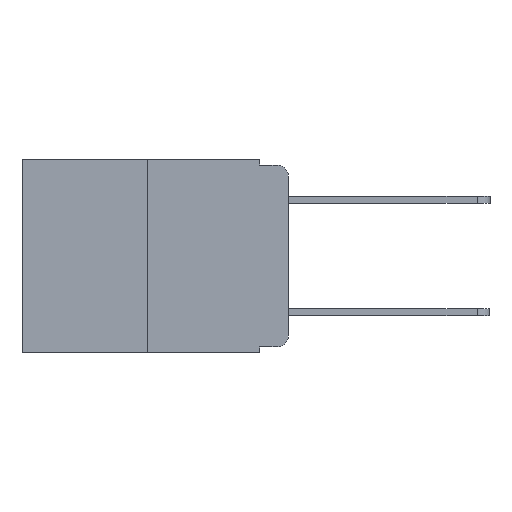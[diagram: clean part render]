
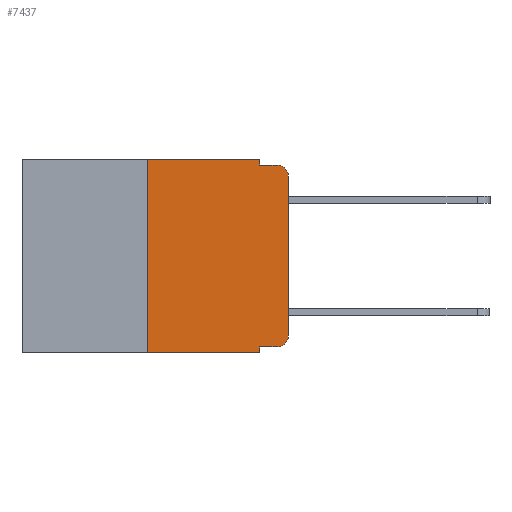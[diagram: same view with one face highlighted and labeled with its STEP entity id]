
A CAD part, left-side view. The second image highlights one B-rep face of the part: STEP entity #7437.
In plain terms, the highlighted planar face has unit normal (-1, 0, 0).
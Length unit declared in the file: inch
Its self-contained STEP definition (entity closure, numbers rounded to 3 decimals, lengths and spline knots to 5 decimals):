
#278 = PLANE ( 'NONE',  #517 ) ;
#517 = AXIS2_PLACEMENT_3D ( 'NONE', #5071, #8735, #3286 ) ;
#566 = ORIENTED_EDGE ( 'NONE', *, *, #10424, .F. ) ;
#667 = VECTOR ( 'NONE', #9923, 39.37008 ) ;
#811 = VERTEX_POINT ( 'NONE', #3382 ) ;
#826 = EDGE_CURVE ( 'NONE', #2921, #2967, #3867, .T. ) ;
#995 = EDGE_CURVE ( 'NONE', #6220, #811, #9644, .T. ) ;
#1177 = EDGE_CURVE ( 'NONE', #3896, #2921, #6181, .T. ) ;
#1472 = CIRCLE ( 'NONE', #2716, 0.02 ) ;
#1535 = CARTESIAN_POINT ( 'NONE',  ( 0., 0.051, -0.333 ) ) ;
#1595 = VERTEX_POINT ( 'NONE', #4728 ) ;
#1749 = EDGE_CURVE ( 'NONE', #9573, #2967, #1472, .T. ) ;
#1868 = ORIENTED_EDGE ( 'NONE', *, *, #7618, .T. ) ;
#2366 = LINE ( 'NONE', #7528, #11412 ) ;
#2716 = AXIS2_PLACEMENT_3D ( 'NONE', #8193, #8180, #8163 ) ;
#2833 = VECTOR ( 'NONE', #5052, 39.37008 ) ;
#2921 = VERTEX_POINT ( 'NONE', #9725 ) ;
#2967 = VERTEX_POINT ( 'NONE', #3908 ) ;
#3044 = VECTOR ( 'NONE', #11447, 39.37008 ) ;
#3098 = VERTEX_POINT ( 'NONE', #3854 ) ;
#3162 = CARTESIAN_POINT ( 'NONE',  ( 0., 0.02, -0.333 ) ) ;
#3228 = CARTESIAN_POINT ( 'NONE',  ( 0., 0.051, 0. ) ) ;
#3286 = DIRECTION ( 'NONE',  ( 0., 0., -1. ) ) ;
#3382 = CARTESIAN_POINT ( 'NONE',  ( 0., 0., -0.313 ) ) ;
#3604 = VECTOR ( 'NONE', #7112, 39.37008 ) ;
#3732 = VECTOR ( 'NONE', #9950, 39.37008 ) ;
#3854 = CARTESIAN_POINT ( 'NONE',  ( 0., 0.25, -0.343 ) ) ;
#3867 = LINE ( 'NONE', #4422, #3604 ) ;
#3881 = LINE ( 'NONE', #10003, #8457 ) ;
#3896 = VERTEX_POINT ( 'NONE', #4019 ) ;
#3908 = CARTESIAN_POINT ( 'NONE',  ( 0., 0.02, -0.01 ) ) ;
#3960 = EDGE_CURVE ( 'NONE', #1595, #3896, #2366, .T. ) ;
#4019 = CARTESIAN_POINT ( 'NONE',  ( 0., 0.051, 0. ) ) ;
#4341 = ORIENTED_EDGE ( 'NONE', *, *, #1749, .T. ) ;
#4422 = CARTESIAN_POINT ( 'NONE',  ( 0., 0.051, -0.01 ) ) ;
#4728 = CARTESIAN_POINT ( 'NONE',  ( 0., 0.25, 0. ) ) ;
#4934 = ORIENTED_EDGE ( 'NONE', *, *, #3960, .F. ) ;
#5052 = DIRECTION ( 'NONE',  ( 0., 0., -1. ) ) ;
#5061 = EDGE_CURVE ( 'NONE', #5370, #6220, #6052, .T. ) ;
#5071 = CARTESIAN_POINT ( 'NONE',  ( 0., 0.473, 0. ) ) ;
#5370 = VERTEX_POINT ( 'NONE', #1535 ) ;
#5424 = CARTESIAN_POINT ( 'NONE',  ( 0., 0.473, -0.343 ) ) ;
#5436 = DIRECTION ( 'NONE',  ( -1., 0., 0. ) ) ;
#5847 = EDGE_LOOP ( 'NONE', ( #1868, #4341, #7118, #11511, #4934, #7663, #7793, #566, #10294, #10787 ) ) ;
#5908 = CARTESIAN_POINT ( 'NONE',  ( 0., 0., -0.03 ) ) ;
#5923 = FACE_OUTER_BOUND ( 'NONE', #5847, .T. ) ;
#6052 = LINE ( 'NONE', #10036, #667 ) ;
#6181 = LINE ( 'NONE', #9910, #3732 ) ;
#6220 = VERTEX_POINT ( 'NONE', #3162 ) ;
#6535 = DIRECTION ( 'NONE',  ( 0., 0., 1. ) ) ;
#6624 = LINE ( 'NONE', #11411, #3044 ) ;
#6630 = AXIS2_PLACEMENT_3D ( 'NONE', #9594, #5436, #7669 ) ;
#7112 = DIRECTION ( 'NONE',  ( 0., -1., 0. ) ) ;
#7118 = ORIENTED_EDGE ( 'NONE', *, *, #826, .F. ) ;
#7192 = EDGE_CURVE ( 'NONE', #3098, #1595, #3881, .T. ) ;
#7402 = LINE ( 'NONE', #3228, #2833 ) ;
#7437 = ADVANCED_FACE ( 'NONE', ( #5923 ), #278, .F. ) ;
#7528 = CARTESIAN_POINT ( 'NONE',  ( 0., 0.473, 0. ) ) ;
#7618 = EDGE_CURVE ( 'NONE', #811, #9573, #6624, .T. ) ;
#7663 = ORIENTED_EDGE ( 'NONE', *, *, #7192, .F. ) ;
#7669 = DIRECTION ( 'NONE',  ( 0., 0., -1. ) ) ;
#7793 = ORIENTED_EDGE ( 'NONE', *, *, #9298, .T. ) ;
#8163 = DIRECTION ( 'NONE',  ( 0., 0., -1. ) ) ;
#8180 = DIRECTION ( 'NONE',  ( -1., 0., 0. ) ) ;
#8193 = CARTESIAN_POINT ( 'NONE',  ( 0., 0.02, -0.03 ) ) ;
#8457 = VECTOR ( 'NONE', #6535, 39.37008 ) ;
#8480 = CARTESIAN_POINT ( 'NONE',  ( 0., 0.051, -0.343 ) ) ;
#8487 = VERTEX_POINT ( 'NONE', #8480 ) ;
#8735 = DIRECTION ( 'NONE',  ( 1., 0., 0. ) ) ;
#9298 = EDGE_CURVE ( 'NONE', #3098, #8487, #9846, .T. ) ;
#9573 = VERTEX_POINT ( 'NONE', #5908 ) ;
#9594 = CARTESIAN_POINT ( 'NONE',  ( 0., 0.02, -0.313 ) ) ;
#9644 = CIRCLE ( 'NONE', #6630, 0.02 ) ;
#9725 = CARTESIAN_POINT ( 'NONE',  ( 0., 0.051, -0.01 ) ) ;
#9834 = DIRECTION ( 'NONE',  ( 0., -1., 0. ) ) ;
#9846 = LINE ( 'NONE', #5424, #11634 ) ;
#9910 = CARTESIAN_POINT ( 'NONE',  ( 0., 0.051, 0. ) ) ;
#9923 = DIRECTION ( 'NONE',  ( 0., -1., 0. ) ) ;
#9950 = DIRECTION ( 'NONE',  ( 0., 0., -1. ) ) ;
#10003 = CARTESIAN_POINT ( 'NONE',  ( 0., 0.25, 0. ) ) ;
#10036 = CARTESIAN_POINT ( 'NONE',  ( 0., 0.051, -0.333 ) ) ;
#10092 = DIRECTION ( 'NONE',  ( 0., -1., 0. ) ) ;
#10294 = ORIENTED_EDGE ( 'NONE', *, *, #5061, .T. ) ;
#10424 = EDGE_CURVE ( 'NONE', #5370, #8487, #7402, .T. ) ;
#10787 = ORIENTED_EDGE ( 'NONE', *, *, #995, .T. ) ;
#11411 = CARTESIAN_POINT ( 'NONE',  ( 0., 0., 0. ) ) ;
#11412 = VECTOR ( 'NONE', #10092, 39.37008 ) ;
#11447 = DIRECTION ( 'NONE',  ( 0., 0., 1. ) ) ;
#11511 = ORIENTED_EDGE ( 'NONE', *, *, #1177, .F. ) ;
#11634 = VECTOR ( 'NONE', #9834, 39.37008 ) ;
